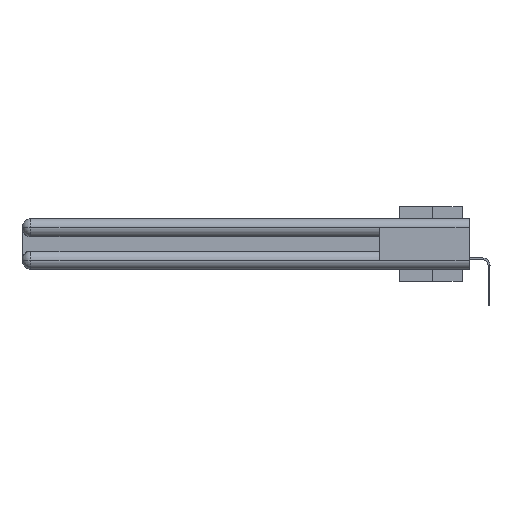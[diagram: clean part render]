
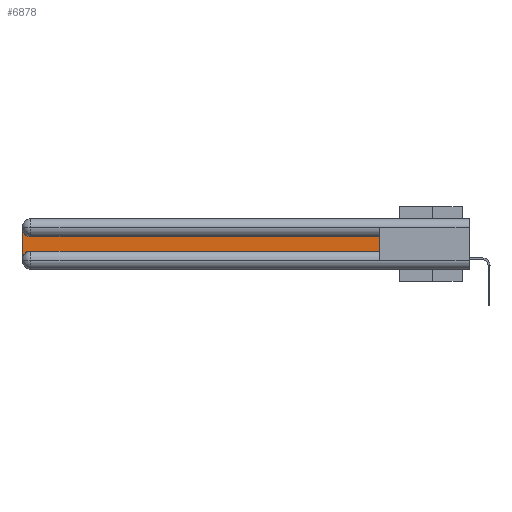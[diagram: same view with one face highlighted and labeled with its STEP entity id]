
A CAD part, left-side view. The second image highlights one B-rep face of the part: STEP entity #6878.
In plain terms, the highlighted planar face has unit normal (-1, 0, 0).
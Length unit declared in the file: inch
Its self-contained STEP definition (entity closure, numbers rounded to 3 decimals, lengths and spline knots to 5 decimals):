
#822 = CARTESIAN_POINT ( 'NONE',  ( 0.075, 0.6, -0.2175 ) ) ;
#1430 = LINE ( 'NONE', #27357, #15629 ) ;
#1661 = DIRECTION ( 'NONE',  ( 0., -1., 0. ) ) ;
#2039 = CIRCLE ( 'NONE', #7197, 0.06 ) ;
#2158 = LINE ( 'NONE', #4561, #29239 ) ;
#3520 = ORIENTED_EDGE ( 'NONE', *, *, #20581, .T. ) ;
#3980 = CARTESIAN_POINT ( 'NONE',  ( 0.075, 3., -0.2775 ) ) ;
#4443 = ORIENTED_EDGE ( 'NONE', *, *, #19559, .T. ) ;
#4561 = CARTESIAN_POINT ( 'NONE',  ( 0.075, 0.6, -0.1225 ) ) ;
#5707 = VERTEX_POINT ( 'NONE', #7170 ) ;
#6878 = ADVANCED_FACE ( 'NONE', ( #30539 ), #28334, .F. ) ;
#7170 = CARTESIAN_POINT ( 'NONE',  ( 0.075, 3., -0.0625 ) ) ;
#7197 = AXIS2_PLACEMENT_3D ( 'NONE', #28912, #28791, #31739 ) ;
#7378 = CARTESIAN_POINT ( 'NONE',  ( 0.075, 2.94, -0.0625 ) ) ;
#9700 = DIRECTION ( 'NONE',  ( 0., 0., 1. ) ) ;
#10606 = DIRECTION ( 'NONE',  ( 0., 1., 0. ) ) ;
#12932 = VERTEX_POINT ( 'NONE', #31979 ) ;
#13084 = CARTESIAN_POINT ( 'NONE',  ( 0.075, 3., -0.1225 ) ) ;
#13645 = ORIENTED_EDGE ( 'NONE', *, *, #29451, .T. ) ;
#14554 = CARTESIAN_POINT ( 'NONE',  ( 0.075, 0.6, -0.2175 ) ) ;
#14657 = VERTEX_POINT ( 'NONE', #14554 ) ;
#15629 = VECTOR ( 'NONE', #15703, 39.37008 ) ;
#15703 = DIRECTION ( 'NONE',  ( 0., 0., -1. ) ) ;
#15792 = EDGE_CURVE ( 'NONE', #22602, #31138, #2158, .T. ) ;
#16386 = VECTOR ( 'NONE', #1661, 39.37008 ) ;
#18343 = VERTEX_POINT ( 'NONE', #3980 ) ;
#18580 = CARTESIAN_POINT ( 'NONE',  ( 0.075, 2.94, -0.1225 ) ) ;
#18793 = DIRECTION ( 'NONE',  ( 1., 0., 0. ) ) ;
#19098 = DIRECTION ( 'NONE',  ( 0., 0., -1. ) ) ;
#19559 = EDGE_CURVE ( 'NONE', #5707, #18343, #1430, .T. ) ;
#20581 = EDGE_CURVE ( 'NONE', #31138, #5707, #28424, .T. ) ;
#22602 = VERTEX_POINT ( 'NONE', #32886 ) ;
#23044 = EDGE_CURVE ( 'NONE', #18343, #12932, #2039, .T. ) ;
#24776 = AXIS2_PLACEMENT_3D ( 'NONE', #13084, #33583, #19098 ) ;
#25050 = DIRECTION ( 'NONE',  ( 0., 0., -1. ) ) ;
#25454 = EDGE_CURVE ( 'NONE', #12932, #14657, #31996, .T. ) ;
#26064 = ORIENTED_EDGE ( 'NONE', *, *, #15792, .T. ) ;
#26467 = ORIENTED_EDGE ( 'NONE', *, *, #25454, .T. ) ;
#27357 = CARTESIAN_POINT ( 'NONE',  ( 0.075, 3., -0.2175 ) ) ;
#27612 = EDGE_LOOP ( 'NONE', ( #26064, #3520, #4443, #27826, #26467, #13645 ) ) ;
#27826 = ORIENTED_EDGE ( 'NONE', *, *, #23044, .T. ) ;
#28334 = PLANE ( 'NONE',  #24776 ) ;
#28424 = CIRCLE ( 'NONE', #30730, 0.06 ) ;
#28791 = DIRECTION ( 'NONE',  ( 1., 0., 0. ) ) ;
#28912 = CARTESIAN_POINT ( 'NONE',  ( 0.075, 2.94, -0.2775 ) ) ;
#29239 = VECTOR ( 'NONE', #10606, 39.37008 ) ;
#29451 = EDGE_CURVE ( 'NONE', #14657, #22602, #37472, .T. ) ;
#30539 = FACE_OUTER_BOUND ( 'NONE', #27612, .T. ) ;
#30730 = AXIS2_PLACEMENT_3D ( 'NONE', #7378, #18793, #25050 ) ;
#31138 = VERTEX_POINT ( 'NONE', #18580 ) ;
#31739 = DIRECTION ( 'NONE',  ( 0., 0., -1. ) ) ;
#31979 = CARTESIAN_POINT ( 'NONE',  ( 0.075, 2.94, -0.2175 ) ) ;
#31996 = LINE ( 'NONE', #36666, #16386 ) ;
#32886 = CARTESIAN_POINT ( 'NONE',  ( 0.075, 0.6, -0.1225 ) ) ;
#33583 = DIRECTION ( 'NONE',  ( 1., 0., 0. ) ) ;
#35137 = VECTOR ( 'NONE', #9700, 39.37008 ) ;
#36666 = CARTESIAN_POINT ( 'NONE',  ( 0.075, 0.6, -0.2175 ) ) ;
#37472 = LINE ( 'NONE', #822, #35137 ) ;
